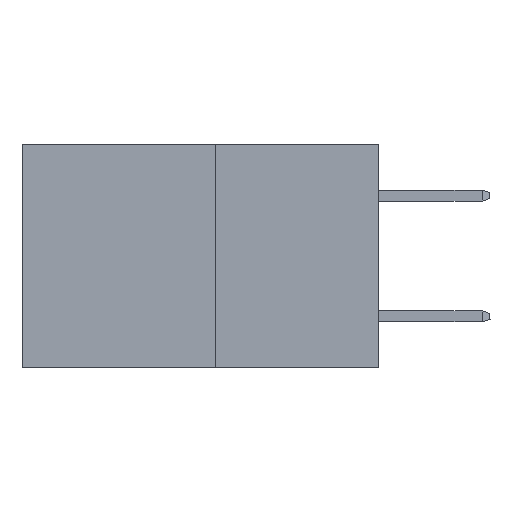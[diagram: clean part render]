
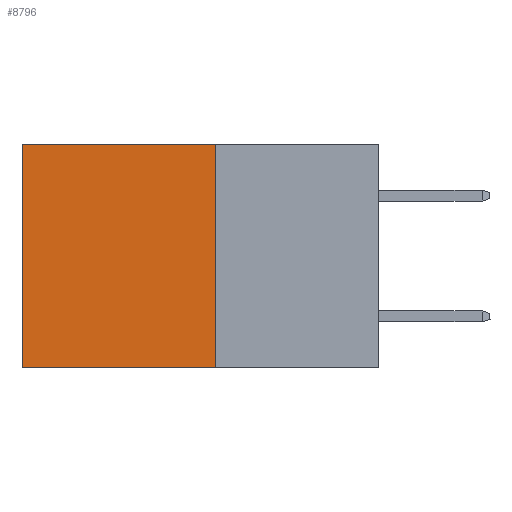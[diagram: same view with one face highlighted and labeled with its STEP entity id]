
A CAD part, left-side view. The second image highlights one B-rep face of the part: STEP entity #8796.
In plain terms, the highlighted planar face has unit normal (-1, 0, 0).
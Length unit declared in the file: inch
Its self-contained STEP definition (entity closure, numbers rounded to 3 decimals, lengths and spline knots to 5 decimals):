
#273 = AXIS2_PLACEMENT_3D ( 'NONE', #9977, #9820, #9749 ) ;
#475 = CARTESIAN_POINT ( 'NONE',  ( 0.277, 0.27, -0.37 ) ) ;
#600 = EDGE_LOOP ( 'NONE', ( #18263, #22155, #5472, #21956 ) ) ;
#2829 = VERTEX_POINT ( 'NONE', #4279 ) ;
#3053 = VERTEX_POINT ( 'NONE', #475 ) ;
#3601 = EDGE_CURVE ( 'NONE', #10805, #11057, #4833, .T. ) ;
#4279 = CARTESIAN_POINT ( 'NONE',  ( 0.277, 0.27, 0. ) ) ;
#4833 = LINE ( 'NONE', #13199, #13670 ) ;
#5465 = VECTOR ( 'NONE', #20866, 39.37008 ) ;
#5472 = ORIENTED_EDGE ( 'NONE', *, *, #11003, .F. ) ;
#6151 = EDGE_CURVE ( 'NONE', #2829, #10805, #12713, .T. ) ;
#6159 = CARTESIAN_POINT ( 'NONE',  ( 0.277, 0.59, 0. ) ) ;
#6540 = VECTOR ( 'NONE', #17798, 39.37008 ) ;
#8022 = VECTOR ( 'NONE', #19333, 39.37008 ) ;
#8796 = ADVANCED_FACE ( 'NONE', ( #14608 ), #10136, .F. ) ;
#9749 = DIRECTION ( 'NONE',  ( 0., 0., -1. ) ) ;
#9820 = DIRECTION ( 'NONE',  ( 1., 0., 0. ) ) ;
#9977 = CARTESIAN_POINT ( 'NONE',  ( 0.277, 0.27, -0.37 ) ) ;
#10136 = PLANE ( 'NONE',  #273 ) ;
#10805 = VERTEX_POINT ( 'NONE', #6159 ) ;
#11003 = EDGE_CURVE ( 'NONE', #2829, #3053, #19508, .T. ) ;
#11057 = VERTEX_POINT ( 'NONE', #13949 ) ;
#11909 = EDGE_CURVE ( 'NONE', #3053, #11057, #15887, .T. ) ;
#12713 = LINE ( 'NONE', #19354, #8022 ) ;
#13199 = CARTESIAN_POINT ( 'NONE',  ( 0.277, 0.59, -0.37 ) ) ;
#13670 = VECTOR ( 'NONE', #14208, 39.37008 ) ;
#13949 = CARTESIAN_POINT ( 'NONE',  ( 0.277, 0.59, -0.37 ) ) ;
#14208 = DIRECTION ( 'NONE',  ( 0., 0., -1. ) ) ;
#14608 = FACE_OUTER_BOUND ( 'NONE', #600, .T. ) ;
#15887 = LINE ( 'NONE', #16031, #6540 ) ;
#16031 = CARTESIAN_POINT ( 'NONE',  ( 0.277, 0.27, -0.37 ) ) ;
#17798 = DIRECTION ( 'NONE',  ( 0., 1., 0. ) ) ;
#18263 = ORIENTED_EDGE ( 'NONE', *, *, #3601, .T. ) ;
#19087 = CARTESIAN_POINT ( 'NONE',  ( 0.277, 0.27, -0.37 ) ) ;
#19333 = DIRECTION ( 'NONE',  ( 0., 1., 0. ) ) ;
#19354 = CARTESIAN_POINT ( 'NONE',  ( 0.277, 0.27, 0. ) ) ;
#19508 = LINE ( 'NONE', #19087, #5465 ) ;
#20866 = DIRECTION ( 'NONE',  ( 0., 0., -1. ) ) ;
#21956 = ORIENTED_EDGE ( 'NONE', *, *, #6151, .T. ) ;
#22155 = ORIENTED_EDGE ( 'NONE', *, *, #11909, .F. ) ;
